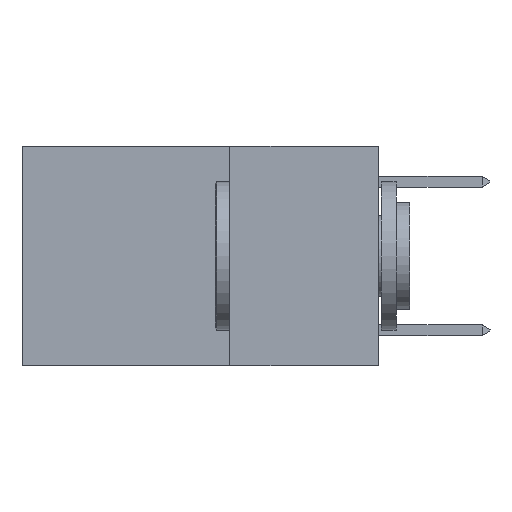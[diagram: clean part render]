
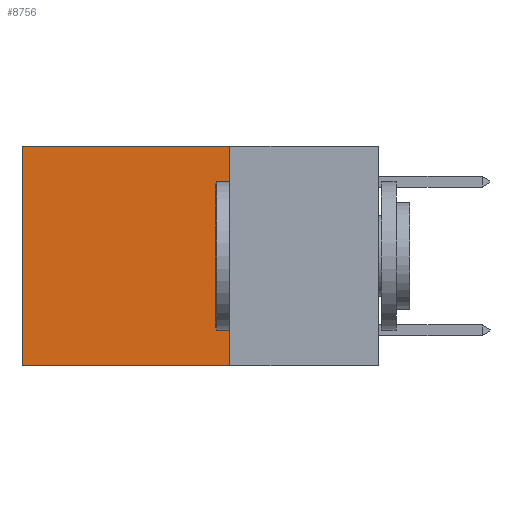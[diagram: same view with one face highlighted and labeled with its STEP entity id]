
A CAD part, left-side view. The second image highlights one B-rep face of the part: STEP entity #8756.
In plain terms, the highlighted planar face has unit normal (-1, 0, 0).
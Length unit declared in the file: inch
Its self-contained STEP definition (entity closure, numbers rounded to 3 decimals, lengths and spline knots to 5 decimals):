
#115 = ORIENTED_EDGE ( 'NONE', *, *, #6430, .T. ) ;
#557 = CARTESIAN_POINT ( 'NONE',  ( 0.2625, 0.25, -0.37 ) ) ;
#785 = DIRECTION ( 'NONE',  ( 0., 0., -1. ) ) ;
#1167 = VECTOR ( 'NONE', #7226, 39.37008 ) ;
#1452 = EDGE_CURVE ( 'NONE', #7710, #3665, #9260, .T. ) ;
#1844 = EDGE_CURVE ( 'NONE', #8954, #5201, #7300, .T. ) ;
#3071 = VECTOR ( 'NONE', #7388, 39.37008 ) ;
#3152 = EDGE_CURVE ( 'NONE', #5201, #3665, #5196, .T. ) ;
#3205 = CARTESIAN_POINT ( 'NONE',  ( 0.2625, 0.6, -0.37 ) ) ;
#3665 = VERTEX_POINT ( 'NONE', #3205 ) ;
#4991 = VECTOR ( 'NONE', #10042, 39.37008 ) ;
#5175 = CARTESIAN_POINT ( 'NONE',  ( 0.2625, 0.25, 0. ) ) ;
#5196 = LINE ( 'NONE', #7626, #3071 ) ;
#5201 = VERTEX_POINT ( 'NONE', #557 ) ;
#5234 = VECTOR ( 'NONE', #7712, 39.37008 ) ;
#5636 = DIRECTION ( 'NONE',  ( 1., 0., 0. ) ) ;
#6210 = CARTESIAN_POINT ( 'NONE',  ( 0.2625, 0.6, 0. ) ) ;
#6430 = EDGE_CURVE ( 'NONE', #8954, #7710, #9473, .T. ) ;
#6735 = AXIS2_PLACEMENT_3D ( 'NONE', #7905, #5636, #785 ) ;
#7226 = DIRECTION ( 'NONE',  ( 0., 1., 0. ) ) ;
#7300 = LINE ( 'NONE', #8488, #5234 ) ;
#7388 = DIRECTION ( 'NONE',  ( 0., 1., 0. ) ) ;
#7529 = EDGE_LOOP ( 'NONE', ( #9232, #9305, #9851, #115 ) ) ;
#7626 = CARTESIAN_POINT ( 'NONE',  ( 0.2625, 0.25, -0.37 ) ) ;
#7710 = VERTEX_POINT ( 'NONE', #8317 ) ;
#7712 = DIRECTION ( 'NONE',  ( 0., 0., -1. ) ) ;
#7905 = CARTESIAN_POINT ( 'NONE',  ( 0.2625, 0.25, 0. ) ) ;
#8061 = FACE_OUTER_BOUND ( 'NONE', #7529, .T. ) ;
#8317 = CARTESIAN_POINT ( 'NONE',  ( 0.2625, 0.6, 0. ) ) ;
#8488 = CARTESIAN_POINT ( 'NONE',  ( 0.2625, 0.25, 0. ) ) ;
#8756 = ADVANCED_FACE ( 'NONE', ( #8061 ), #9369, .F. ) ;
#8954 = VERTEX_POINT ( 'NONE', #5175 ) ;
#9232 = ORIENTED_EDGE ( 'NONE', *, *, #1452, .T. ) ;
#9260 = LINE ( 'NONE', #6210, #4991 ) ;
#9305 = ORIENTED_EDGE ( 'NONE', *, *, #3152, .F. ) ;
#9369 = PLANE ( 'NONE',  #6735 ) ;
#9404 = CARTESIAN_POINT ( 'NONE',  ( 0.2625, 0.25, 0. ) ) ;
#9473 = LINE ( 'NONE', #9404, #1167 ) ;
#9851 = ORIENTED_EDGE ( 'NONE', *, *, #1844, .F. ) ;
#10042 = DIRECTION ( 'NONE',  ( 0., 0., -1. ) ) ;
